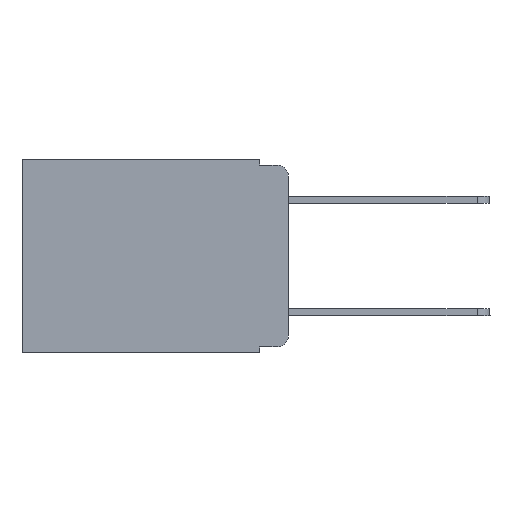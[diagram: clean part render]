
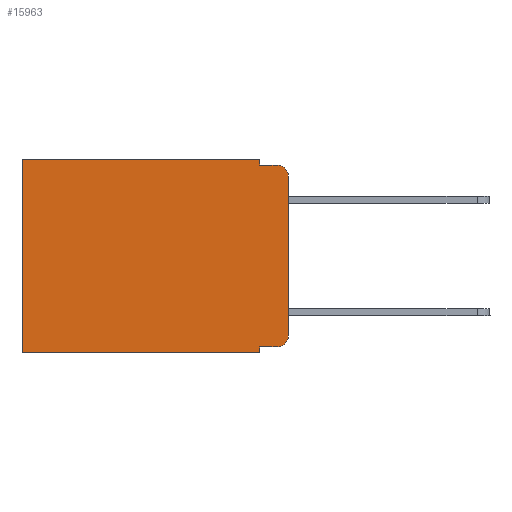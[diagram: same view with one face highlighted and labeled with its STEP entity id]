
A CAD part, left-side view. The second image highlights one B-rep face of the part: STEP entity #15963.
In plain terms, the highlighted planar face has unit normal (-1, 0, 0).
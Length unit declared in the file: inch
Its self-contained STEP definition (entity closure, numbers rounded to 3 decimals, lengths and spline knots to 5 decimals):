
#24 = ORIENTED_EDGE ( 'NONE', *, *, #14870, .F. ) ;
#133 = DIRECTION ( 'NONE',  ( 0., 0., -1. ) ) ;
#376 = CARTESIAN_POINT ( 'NONE',  ( 0.298, 0.473, 0. ) ) ;
#749 = CARTESIAN_POINT ( 'NONE',  ( 0.298, 0., -0.343 ) ) ;
#838 = EDGE_LOOP ( 'NONE', ( #24, #15680, #15697, #1973, #12047, #9494, #7430, #12010, #12078, #3377 ) ) ;
#1487 = EDGE_CURVE ( 'NONE', #10668, #13186, #10602, .T. ) ;
#1599 = CARTESIAN_POINT ( 'NONE',  ( 0.298, 0.02, -0.313 ) ) ;
#1766 = EDGE_CURVE ( 'NONE', #2298, #11384, #10173, .T. ) ;
#1973 = ORIENTED_EDGE ( 'NONE', *, *, #13679, .F. ) ;
#2240 = AXIS2_PLACEMENT_3D ( 'NONE', #7473, #7794, #7713 ) ;
#2298 = VERTEX_POINT ( 'NONE', #9255 ) ;
#2359 = CARTESIAN_POINT ( 'NONE',  ( 0.298, 0.051, -0.01 ) ) ;
#2668 = EDGE_CURVE ( 'NONE', #5136, #11384, #11314, .T. ) ;
#3037 = CARTESIAN_POINT ( 'NONE',  ( 0.298, 0.051, -0.333 ) ) ;
#3186 = AXIS2_PLACEMENT_3D ( 'NONE', #12198, #3649, #6041 ) ;
#3264 = EDGE_CURVE ( 'NONE', #13254, #8824, #3892, .T. ) ;
#3377 = ORIENTED_EDGE ( 'NONE', *, *, #3264, .T. ) ;
#3577 = FACE_OUTER_BOUND ( 'NONE', #838, .T. ) ;
#3649 = DIRECTION ( 'NONE',  ( 1., 0., 0. ) ) ;
#3717 = EDGE_CURVE ( 'NONE', #15256, #13254, #13239, .T. ) ;
#3832 = EDGE_CURVE ( 'NONE', #9314, #10668, #9498, .T. ) ;
#3892 = CIRCLE ( 'NONE', #14213, 0.02 ) ;
#4319 = VERTEX_POINT ( 'NONE', #6229 ) ;
#4470 = DIRECTION ( 'NONE',  ( -1., 0., 0. ) ) ;
#4699 = CARTESIAN_POINT ( 'NONE',  ( 0.298, 0.051, 0. ) ) ;
#4931 = VECTOR ( 'NONE', #6416, 39.37008 ) ;
#5136 = VERTEX_POINT ( 'NONE', #2359 ) ;
#5406 = VECTOR ( 'NONE', #7975, 39.37008 ) ;
#6041 = DIRECTION ( 'NONE',  ( 0., 0., -1. ) ) ;
#6229 = CARTESIAN_POINT ( 'NONE',  ( 0.298, 0.051, -0.343 ) ) ;
#6416 = DIRECTION ( 'NONE',  ( 0., -1., 0. ) ) ;
#6688 = DIRECTION ( 'NONE',  ( 0., -1., 0. ) ) ;
#6730 = CARTESIAN_POINT ( 'NONE',  ( 0.298, 0.02, -0.01 ) ) ;
#6833 = EDGE_CURVE ( 'NONE', #15256, #4319, #13684, .T. ) ;
#7430 = ORIENTED_EDGE ( 'NONE', *, *, #15231, .F. ) ;
#7473 = CARTESIAN_POINT ( 'NONE',  ( 0.298, 0.02, -0.03 ) ) ;
#7713 = DIRECTION ( 'NONE',  ( 0., 0., -1. ) ) ;
#7794 = DIRECTION ( 'NONE',  ( -1., 0., 0. ) ) ;
#7975 = DIRECTION ( 'NONE',  ( 0., 0., -1. ) ) ;
#8824 = VERTEX_POINT ( 'NONE', #14910 ) ;
#9081 = CARTESIAN_POINT ( 'NONE',  ( 0.298, 0.051, -0.333 ) ) ;
#9255 = CARTESIAN_POINT ( 'NONE',  ( 0.298, 0., -0.03 ) ) ;
#9314 = VERTEX_POINT ( 'NONE', #4699 ) ;
#9444 = VECTOR ( 'NONE', #9819, 39.37008 ) ;
#9494 = ORIENTED_EDGE ( 'NONE', *, *, #1487, .T. ) ;
#9498 = LINE ( 'NONE', #9740, #9444 ) ;
#9668 = CARTESIAN_POINT ( 'NONE',  ( 0.298, 0.02, -0.333 ) ) ;
#9740 = CARTESIAN_POINT ( 'NONE',  ( 0.298, 0., 0. ) ) ;
#9769 = VECTOR ( 'NONE', #14844, 39.37008 ) ;
#9819 = DIRECTION ( 'NONE',  ( 0., 1., 0. ) ) ;
#10173 = CIRCLE ( 'NONE', #2240, 0.02 ) ;
#10602 = LINE ( 'NONE', #376, #5406 ) ;
#10668 = VERTEX_POINT ( 'NONE', #10726 ) ;
#10726 = CARTESIAN_POINT ( 'NONE',  ( 0.298, 0.473, 0. ) ) ;
#10791 = DIRECTION ( 'NONE',  ( 0., 0., -1. ) ) ;
#10818 = CARTESIAN_POINT ( 'NONE',  ( 0.298, 0.473, -0.343 ) ) ;
#11314 = LINE ( 'NONE', #15063, #4931 ) ;
#11384 = VERTEX_POINT ( 'NONE', #6730 ) ;
#12010 = ORIENTED_EDGE ( 'NONE', *, *, #6833, .F. ) ;
#12047 = ORIENTED_EDGE ( 'NONE', *, *, #3832, .T. ) ;
#12078 = ORIENTED_EDGE ( 'NONE', *, *, #3717, .T. ) ;
#12198 = CARTESIAN_POINT ( 'NONE',  ( 0.298, 0., 0. ) ) ;
#12455 = DIRECTION ( 'NONE',  ( 0., 0., -1. ) ) ;
#12758 = VECTOR ( 'NONE', #12455, 39.37008 ) ;
#13182 = VECTOR ( 'NONE', #10791, 39.37008 ) ;
#13186 = VERTEX_POINT ( 'NONE', #10818 ) ;
#13239 = LINE ( 'NONE', #3037, #15291 ) ;
#13254 = VERTEX_POINT ( 'NONE', #9668 ) ;
#13311 = CARTESIAN_POINT ( 'NONE',  ( 0.298, 0.051, 0. ) ) ;
#13609 = CARTESIAN_POINT ( 'NONE',  ( 0.298, 0.051, 0. ) ) ;
#13679 = EDGE_CURVE ( 'NONE', #9314, #5136, #14477, .T. ) ;
#13684 = LINE ( 'NONE', #13609, #12758 ) ;
#13759 = DIRECTION ( 'NONE',  ( 0., 0., -1. ) ) ;
#13760 = PLANE ( 'NONE',  #3186 ) ;
#14213 = AXIS2_PLACEMENT_3D ( 'NONE', #1599, #4470, #133 ) ;
#14477 = LINE ( 'NONE', #13311, #13182 ) ;
#14816 = VECTOR ( 'NONE', #13759, 39.37008 ) ;
#14844 = DIRECTION ( 'NONE',  ( 0., 1., 0. ) ) ;
#14870 = EDGE_CURVE ( 'NONE', #2298, #8824, #15431, .T. ) ;
#14910 = CARTESIAN_POINT ( 'NONE',  ( 0.298, 0., -0.313 ) ) ;
#15063 = CARTESIAN_POINT ( 'NONE',  ( 0.298, 0.051, -0.01 ) ) ;
#15231 = EDGE_CURVE ( 'NONE', #4319, #13186, #15909, .T. ) ;
#15256 = VERTEX_POINT ( 'NONE', #9081 ) ;
#15291 = VECTOR ( 'NONE', #6688, 39.37008 ) ;
#15431 = LINE ( 'NONE', #16336, #14816 ) ;
#15680 = ORIENTED_EDGE ( 'NONE', *, *, #1766, .T. ) ;
#15697 = ORIENTED_EDGE ( 'NONE', *, *, #2668, .F. ) ;
#15909 = LINE ( 'NONE', #749, #9769 ) ;
#15963 = ADVANCED_FACE ( 'NONE', ( #3577 ), #13760, .F. ) ;
#16336 = CARTESIAN_POINT ( 'NONE',  ( 0.298, 0., 0. ) ) ;
